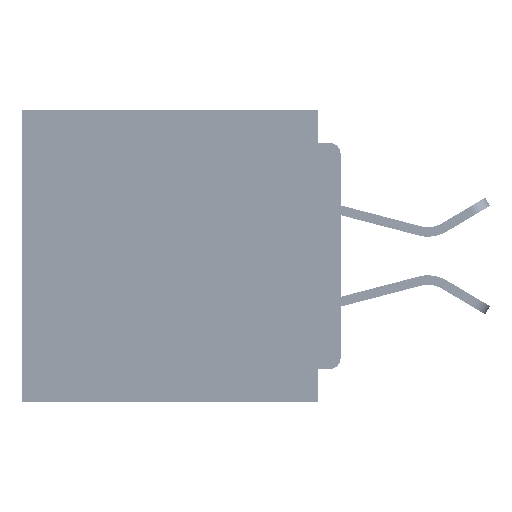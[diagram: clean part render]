
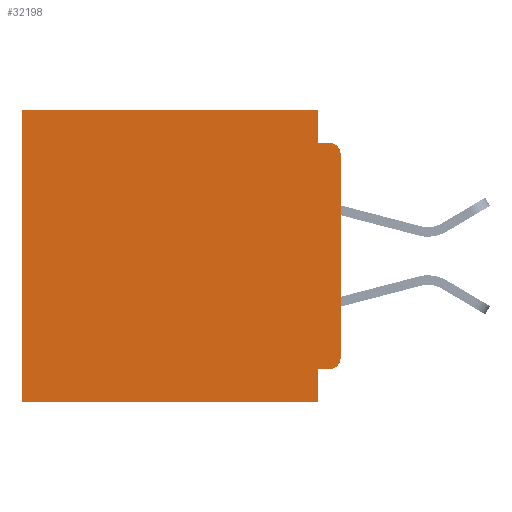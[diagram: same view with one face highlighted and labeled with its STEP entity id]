
A CAD part, left-side view. The second image highlights one B-rep face of the part: STEP entity #32198.
In plain terms, the highlighted planar face has unit normal (-1, 0, 0).
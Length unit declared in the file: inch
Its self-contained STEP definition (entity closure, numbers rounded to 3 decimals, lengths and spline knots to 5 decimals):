
#809 = VERTEX_POINT ( 'NONE', #53358 ) ;
#1854 = CARTESIAN_POINT ( 'NONE',  ( 0.3, 0., -0.06 ) ) ;
#2585 = CARTESIAN_POINT ( 'NONE',  ( 0.3, 0.015, -0.045 ) ) ;
#3853 = PLANE ( 'NONE',  #53132 ) ;
#4076 = VECTOR ( 'NONE', #50971, 39.37008 ) ;
#4234 = CARTESIAN_POINT ( 'NONE',  ( 0.3, 0.437, 0. ) ) ;
#5229 = VECTOR ( 'NONE', #20710, 39.37008 ) ;
#5927 = VECTOR ( 'NONE', #18153, 39.37008 ) ;
#6610 = LINE ( 'NONE', #46806, #5229 ) ;
#6629 = VERTEX_POINT ( 'NONE', #54507 ) ;
#8216 = DIRECTION ( 'NONE',  ( -1., 0., 0. ) ) ;
#8460 = CARTESIAN_POINT ( 'NONE',  ( 0.3, 0.015, -0.355 ) ) ;
#8727 = CARTESIAN_POINT ( 'NONE',  ( 0.3, 0., -0.045 ) ) ;
#8767 = VECTOR ( 'NONE', #36021, 39.37008 ) ;
#9128 = EDGE_CURVE ( 'NONE', #45487, #6629, #52925, .T. ) ;
#10126 = LINE ( 'NONE', #49130, #8767 ) ;
#10967 = EDGE_CURVE ( 'NONE', #19241, #12477, #10126, .T. ) ;
#11063 = LINE ( 'NONE', #50738, #34275 ) ;
#12252 = ORIENTED_EDGE ( 'NONE', *, *, #10967, .F. ) ;
#12377 = LINE ( 'NONE', #8727, #36915 ) ;
#12477 = VERTEX_POINT ( 'NONE', #42019 ) ;
#13062 = AXIS2_PLACEMENT_3D ( 'NONE', #34346, #8216, #38759 ) ;
#18153 = DIRECTION ( 'NONE',  ( 0., 0., -1. ) ) ;
#18814 = CARTESIAN_POINT ( 'NONE',  ( 0.3, 0.031, 0. ) ) ;
#19038 = EDGE_CURVE ( 'NONE', #12477, #38014, #12377, .T. ) ;
#19241 = VERTEX_POINT ( 'NONE', #18814 ) ;
#20264 = DIRECTION ( 'NONE',  ( 0., 1., 0. ) ) ;
#20468 = CARTESIAN_POINT ( 'NONE',  ( 0.3, 0.015, -0.06 ) ) ;
#20494 = CARTESIAN_POINT ( 'NONE',  ( 0.3, 0., 0. ) ) ;
#20710 = DIRECTION ( 'NONE',  ( 0., 0., -1. ) ) ;
#21381 = DIRECTION ( 'NONE',  ( 0., 0., -1. ) ) ;
#21511 = CIRCLE ( 'NONE', #56174, 0.015 ) ;
#22202 = FACE_OUTER_BOUND ( 'NONE', #23797, .T. ) ;
#23309 = EDGE_CURVE ( 'NONE', #38525, #32256, #30553, .T. ) ;
#23797 = EDGE_LOOP ( 'NONE', ( #40646, #43860, #44314, #12252, #52045, #52837, #32109, #33005, #52256, #30697 ) ) ;
#24891 = DIRECTION ( 'NONE',  ( 0., 0., -1. ) ) ;
#26283 = CIRCLE ( 'NONE', #13062, 0.015 ) ;
#28131 = CARTESIAN_POINT ( 'NONE',  ( 0.3, 0.437, -0.4 ) ) ;
#28849 = LINE ( 'NONE', #28131, #36296 ) ;
#28960 = VERTEX_POINT ( 'NONE', #8460 ) ;
#28971 = VERTEX_POINT ( 'NONE', #4234 ) ;
#30553 = LINE ( 'NONE', #39912, #5927 ) ;
#30697 = ORIENTED_EDGE ( 'NONE', *, *, #32586, .T. ) ;
#31447 = EDGE_CURVE ( 'NONE', #809, #45487, #6610, .T. ) ;
#32109 = ORIENTED_EDGE ( 'NONE', *, *, #9128, .F. ) ;
#32198 = ADVANCED_FACE ( 'NONE', ( #22202 ), #3853, .F. ) ;
#32256 = VERTEX_POINT ( 'NONE', #47858 ) ;
#32586 = EDGE_CURVE ( 'NONE', #28960, #32256, #26283, .T. ) ;
#33005 = ORIENTED_EDGE ( 'NONE', *, *, #31447, .F. ) ;
#34275 = VECTOR ( 'NONE', #20264, 39.37008 ) ;
#34346 = CARTESIAN_POINT ( 'NONE',  ( 0.3, 0.015, -0.34 ) ) ;
#36021 = DIRECTION ( 'NONE',  ( 0., 0., -1. ) ) ;
#36296 = VECTOR ( 'NONE', #49957, 39.37008 ) ;
#36647 = EDGE_CURVE ( 'NONE', #28971, #6629, #28849, .T. ) ;
#36915 = VECTOR ( 'NONE', #39272, 39.37008 ) ;
#38014 = VERTEX_POINT ( 'NONE', #2585 ) ;
#38525 = VERTEX_POINT ( 'NONE', #1854 ) ;
#38706 = EDGE_CURVE ( 'NONE', #19241, #28971, #49076, .T. ) ;
#38759 = DIRECTION ( 'NONE',  ( 0., 0., -1. ) ) ;
#38797 = CARTESIAN_POINT ( 'NONE',  ( 0.3, 0., -0.4 ) ) ;
#39272 = DIRECTION ( 'NONE',  ( 0., -1., 0. ) ) ;
#39912 = CARTESIAN_POINT ( 'NONE',  ( 0.3, 0., -0.4 ) ) ;
#40646 = ORIENTED_EDGE ( 'NONE', *, *, #23309, .F. ) ;
#41382 = CARTESIAN_POINT ( 'NONE',  ( 0.3, 0., -0.4 ) ) ;
#42019 = CARTESIAN_POINT ( 'NONE',  ( 0.3, 0.031, -0.045 ) ) ;
#43860 = ORIENTED_EDGE ( 'NONE', *, *, #44211, .T. ) ;
#44211 = EDGE_CURVE ( 'NONE', #38525, #38014, #21511, .T. ) ;
#44314 = ORIENTED_EDGE ( 'NONE', *, *, #19038, .F. ) ;
#45487 = VERTEX_POINT ( 'NONE', #50995 ) ;
#46806 = CARTESIAN_POINT ( 'NONE',  ( 0.3, 0.031, -0.4 ) ) ;
#47490 = DIRECTION ( 'NONE',  ( 1., 0., 0. ) ) ;
#47858 = CARTESIAN_POINT ( 'NONE',  ( 0.3, 0., -0.34 ) ) ;
#49076 = LINE ( 'NONE', #20494, #4076 ) ;
#49130 = CARTESIAN_POINT ( 'NONE',  ( 0.3, 0.031, 0. ) ) ;
#49957 = DIRECTION ( 'NONE',  ( 0., 0., -1. ) ) ;
#50738 = CARTESIAN_POINT ( 'NONE',  ( 0.3, 0., -0.355 ) ) ;
#50936 = DIRECTION ( 'NONE',  ( -1., 0., 0. ) ) ;
#50971 = DIRECTION ( 'NONE',  ( 0., 1., 0. ) ) ;
#50995 = CARTESIAN_POINT ( 'NONE',  ( 0.3, 0.031, -0.4 ) ) ;
#51597 = VECTOR ( 'NONE', #54257, 39.37008 ) ;
#52045 = ORIENTED_EDGE ( 'NONE', *, *, #38706, .T. ) ;
#52256 = ORIENTED_EDGE ( 'NONE', *, *, #52928, .F. ) ;
#52837 = ORIENTED_EDGE ( 'NONE', *, *, #36647, .T. ) ;
#52925 = LINE ( 'NONE', #41382, #51597 ) ;
#52928 = EDGE_CURVE ( 'NONE', #28960, #809, #11063, .T. ) ;
#53132 = AXIS2_PLACEMENT_3D ( 'NONE', #38797, #47490, #21381 ) ;
#53358 = CARTESIAN_POINT ( 'NONE',  ( 0.3, 0.031, -0.355 ) ) ;
#54257 = DIRECTION ( 'NONE',  ( 0., 1., 0. ) ) ;
#54507 = CARTESIAN_POINT ( 'NONE',  ( 0.3, 0.437, -0.4 ) ) ;
#56174 = AXIS2_PLACEMENT_3D ( 'NONE', #20468, #50936, #24891 ) ;
